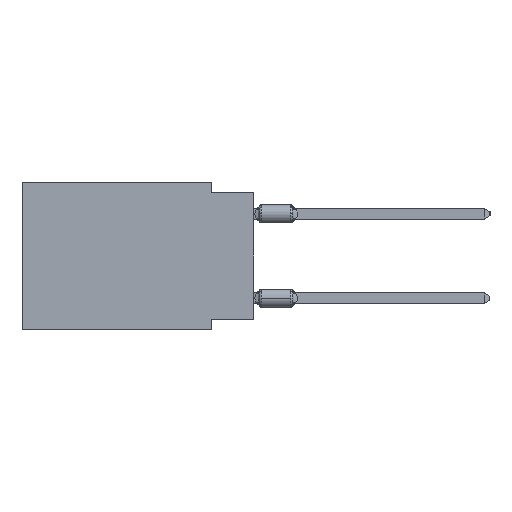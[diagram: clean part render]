
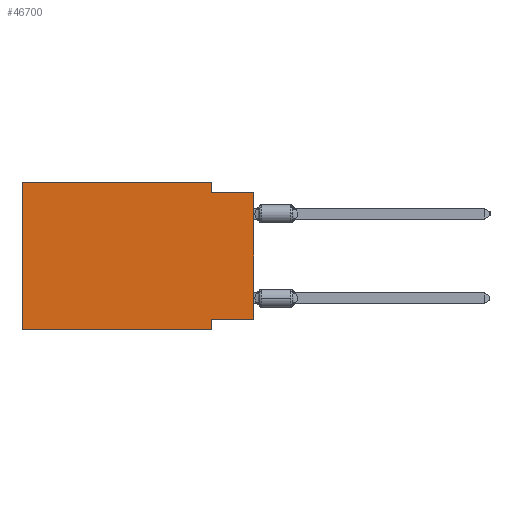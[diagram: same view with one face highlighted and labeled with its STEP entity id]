
A CAD part, left-side view. The second image highlights one B-rep face of the part: STEP entity #46700.
In plain terms, the highlighted planar face has unit normal (-1, 0, 0).
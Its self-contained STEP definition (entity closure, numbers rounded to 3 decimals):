
#347 = EDGE_LOOP ( 'NONE', ( #31861, #16686, #7712, #3176, #39759, #38255, #28602, #30885 ) ) ;
#561 = CARTESIAN_POINT ( 'NONE',  ( 0., 13.97, -8.89 ) ) ;
#700 = EDGE_CURVE ( 'NONE', #20251, #12524, #19310, .T. ) ;
#1476 = LINE ( 'NONE', #27484, #2889 ) ;
#2419 = CARTESIAN_POINT ( 'NONE',  ( 0., 0., 0. ) ) ;
#2843 = PLANE ( 'NONE',  #28640 ) ;
#2889 = VECTOR ( 'NONE', #15926, 1000. ) ;
#3176 = ORIENTED_EDGE ( 'NONE', *, *, #700, .F. ) ;
#4054 = CARTESIAN_POINT ( 'NONE',  ( 0., 0., -8.255 ) ) ;
#4949 = EDGE_CURVE ( 'NONE', #44733, #30642, #30809, .T. ) ;
#6461 = CARTESIAN_POINT ( 'NONE',  ( 0., 13.97, -8.89 ) ) ;
#7203 = DIRECTION ( 'NONE',  ( 0., -1., 0. ) ) ;
#7712 = ORIENTED_EDGE ( 'NONE', *, *, #31812, .F. ) ;
#7782 = CARTESIAN_POINT ( 'NONE',  ( 0., 2.54, 0. ) ) ;
#8936 = CARTESIAN_POINT ( 'NONE',  ( 0., 2.54, 0. ) ) ;
#9805 = VERTEX_POINT ( 'NONE', #41432 ) ;
#11570 = CARTESIAN_POINT ( 'NONE',  ( 0., 13.97, 0. ) ) ;
#11758 = EDGE_CURVE ( 'NONE', #19205, #23911, #27485, .T. ) ;
#11835 = VECTOR ( 'NONE', #16653, 1000. ) ;
#12420 = DIRECTION ( 'NONE',  ( 0., 1., 0. ) ) ;
#12524 = VERTEX_POINT ( 'NONE', #7782 ) ;
#12886 = LINE ( 'NONE', #44790, #35032 ) ;
#15926 = DIRECTION ( 'NONE',  ( 0., 0., -1. ) ) ;
#15934 = CARTESIAN_POINT ( 'NONE',  ( 0., 2.54, -8.255 ) ) ;
#16016 = EDGE_CURVE ( 'NONE', #9805, #23911, #39561, .T. ) ;
#16065 = VECTOR ( 'NONE', #20619, 1000. ) ;
#16311 = EDGE_CURVE ( 'NONE', #21169, #30642, #1476, .T. ) ;
#16653 = DIRECTION ( 'NONE',  ( 0., -1., 0. ) ) ;
#16686 = ORIENTED_EDGE ( 'NONE', *, *, #16016, .F. ) ;
#17375 = CARTESIAN_POINT ( 'NONE',  ( 0., 0., -0.635 ) ) ;
#19205 = VERTEX_POINT ( 'NONE', #4054 ) ;
#19310 = LINE ( 'NONE', #26154, #37971 ) ;
#20251 = VERTEX_POINT ( 'NONE', #11570 ) ;
#20309 = CARTESIAN_POINT ( 'NONE',  ( 0., 0., -0.635 ) ) ;
#20583 = DIRECTION ( 'NONE',  ( 1., 0., 0. ) ) ;
#20619 = DIRECTION ( 'NONE',  ( 0., 0., 1. ) ) ;
#20814 = DIRECTION ( 'NONE',  ( 0., 0., -1. ) ) ;
#21169 = VERTEX_POINT ( 'NONE', #15934 ) ;
#23410 = LINE ( 'NONE', #26730, #40155 ) ;
#23911 = VERTEX_POINT ( 'NONE', #20309 ) ;
#26154 = CARTESIAN_POINT ( 'NONE',  ( 0., 13.97, 0. ) ) ;
#26730 = CARTESIAN_POINT ( 'NONE',  ( 0., 13.97, 0. ) ) ;
#27485 = LINE ( 'NONE', #2419, #16065 ) ;
#27484 = CARTESIAN_POINT ( 'NONE',  ( 0., 2.54, -8.89 ) ) ;
#27888 = VECTOR ( 'NONE', #40841, 1000. ) ;
#27907 = FACE_OUTER_BOUND ( 'NONE', #347, .T. ) ;
#28602 = ORIENTED_EDGE ( 'NONE', *, *, #16311, .F. ) ;
#28640 = AXIS2_PLACEMENT_3D ( 'NONE', #35912, #20583, #20814 ) ;
#29502 = LINE ( 'NONE', #8936, #27888 ) ;
#30642 = VERTEX_POINT ( 'NONE', #38194 ) ;
#30809 = LINE ( 'NONE', #6461, #11835 ) ;
#30885 = ORIENTED_EDGE ( 'NONE', *, *, #39573, .F. ) ;
#31812 = EDGE_CURVE ( 'NONE', #12524, #9805, #29502, .T. ) ;
#31861 = ORIENTED_EDGE ( 'NONE', *, *, #11758, .T. ) ;
#33387 = VECTOR ( 'NONE', #7203, 1000. ) ;
#35032 = VECTOR ( 'NONE', #12420, 1000. ) ;
#35912 = CARTESIAN_POINT ( 'NONE',  ( 0., 13.97, 0. ) ) ;
#37828 = DIRECTION ( 'NONE',  ( 0., 0., 1. ) ) ;
#37909 = EDGE_CURVE ( 'NONE', #44733, #20251, #23410, .T. ) ;
#37971 = VECTOR ( 'NONE', #44597, 1000. ) ;
#38194 = CARTESIAN_POINT ( 'NONE',  ( 0., 2.54, -8.89 ) ) ;
#38255 = ORIENTED_EDGE ( 'NONE', *, *, #4949, .T. ) ;
#39561 = LINE ( 'NONE', #17375, #33387 ) ;
#39573 = EDGE_CURVE ( 'NONE', #19205, #21169, #12886, .T. ) ;
#39759 = ORIENTED_EDGE ( 'NONE', *, *, #37909, .F. ) ;
#40155 = VECTOR ( 'NONE', #37828, 1000. ) ;
#40841 = DIRECTION ( 'NONE',  ( 0., 0., -1. ) ) ;
#41432 = CARTESIAN_POINT ( 'NONE',  ( 0., 2.54, -0.635 ) ) ;
#44597 = DIRECTION ( 'NONE',  ( 0., -1., 0. ) ) ;
#44733 = VERTEX_POINT ( 'NONE', #561 ) ;
#44790 = CARTESIAN_POINT ( 'NONE',  ( 0., 0., -8.255 ) ) ;
#46700 = ADVANCED_FACE ( 'NONE', ( #27907 ), #2843, .F. ) ;
